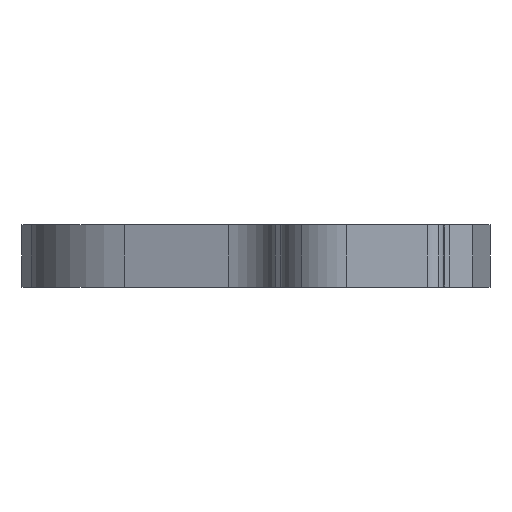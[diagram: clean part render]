
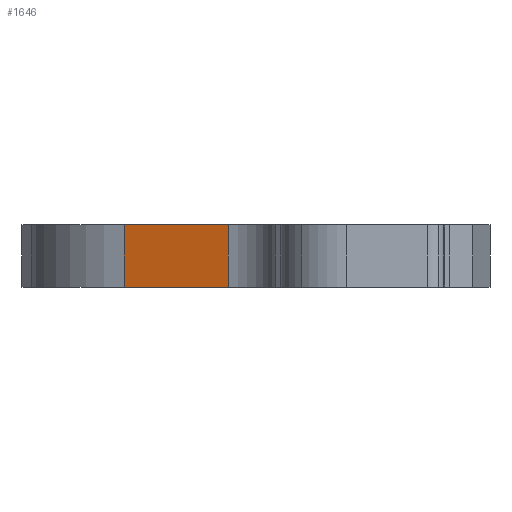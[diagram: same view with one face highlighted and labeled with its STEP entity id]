
A CAD part, left-side view. The second image highlights one B-rep face of the part: STEP entity #1646.
In plain terms, the highlighted planar face has unit normal (-0.958, 0.288, 0).
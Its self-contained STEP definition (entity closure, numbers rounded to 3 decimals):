
#177 = CARTESIAN_POINT ( 'NONE',  ( -9.89, 13.048, 0. ) ) ;
#382 = ORIENTED_EDGE ( 'NONE', *, *, #1153, .F. ) ;
#414 = PLANE ( 'NONE',  #1425 ) ;
#419 = EDGE_CURVE ( 'NONE', #1428, #1549, #1368, .T. ) ;
#446 = ORIENTED_EDGE ( 'NONE', *, *, #609, .F. ) ;
#475 = CARTESIAN_POINT ( 'NONE',  ( -9.89, 13.048, 3. ) ) ;
#479 = LINE ( 'NONE', #999, #1436 ) ;
#501 = ORIENTED_EDGE ( 'NONE', *, *, #1091, .T. ) ;
#539 = CARTESIAN_POINT ( 'NONE',  ( -11.387, 8.076, 0. ) ) ;
#598 = CARTESIAN_POINT ( 'NONE',  ( -11.387, 8.076, 3. ) ) ;
#609 = EDGE_CURVE ( 'NONE', #1428, #1391, #1412, .T. ) ;
#674 = DIRECTION ( 'NONE',  ( 0., 0., 1. ) ) ;
#741 = CARTESIAN_POINT ( 'NONE',  ( -9.89, 13.048, 0. ) ) ;
#889 = ORIENTED_EDGE ( 'NONE', *, *, #419, .T. ) ;
#945 = VERTEX_POINT ( 'NONE', #598 ) ;
#984 = CARTESIAN_POINT ( 'NONE',  ( -9.89, 13.048, 0. ) ) ;
#989 = CARTESIAN_POINT ( 'NONE',  ( -11.387, 8.076, 0. ) ) ;
#999 = CARTESIAN_POINT ( 'NONE',  ( -9.89, 13.048, 3. ) ) ;
#1001 = DIRECTION ( 'NONE',  ( -0.288, -0.958, 0. ) ) ;
#1044 = CARTESIAN_POINT ( 'NONE',  ( -9.89, 13.048, 0. ) ) ;
#1091 = EDGE_CURVE ( 'NONE', #1549, #945, #1116, .T. ) ;
#1096 = VECTOR ( 'NONE', #1001, 1000. ) ;
#1116 = LINE ( 'NONE', #989, #1511 ) ;
#1141 = EDGE_LOOP ( 'NONE', ( #889, #501, #382, #446 ) ) ;
#1142 = DIRECTION ( 'NONE',  ( -0.288, -0.958, 0. ) ) ;
#1153 = EDGE_CURVE ( 'NONE', #1391, #945, #479, .T. ) ;
#1220 = DIRECTION ( 'NONE',  ( 0., 0., 1. ) ) ;
#1368 = LINE ( 'NONE', #741, #1096 ) ;
#1391 = VERTEX_POINT ( 'NONE', #475 ) ;
#1412 = LINE ( 'NONE', #1044, #1513 ) ;
#1425 = AXIS2_PLACEMENT_3D ( 'NONE', #177, #1463, #1220 ) ;
#1428 = VERTEX_POINT ( 'NONE', #984 ) ;
#1436 = VECTOR ( 'NONE', #1142, 1000. ) ;
#1463 = DIRECTION ( 'NONE',  ( -0.958, 0.288, 0. ) ) ;
#1493 = DIRECTION ( 'NONE',  ( 0., 0., 1. ) ) ;
#1511 = VECTOR ( 'NONE', #1493, 1000. ) ;
#1513 = VECTOR ( 'NONE', #674, 1000. ) ;
#1514 = FACE_OUTER_BOUND ( 'NONE', #1141, .T. ) ;
#1549 = VERTEX_POINT ( 'NONE', #539 ) ;
#1646 = ADVANCED_FACE ( 'NONE', ( #1514 ), #414, .T. ) ;
